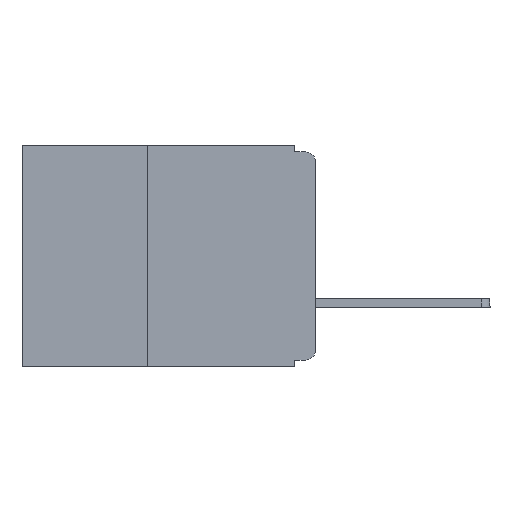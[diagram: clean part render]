
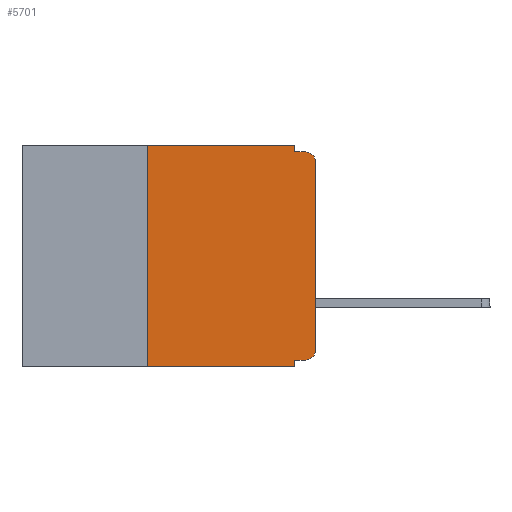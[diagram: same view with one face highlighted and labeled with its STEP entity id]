
A CAD part, left-side view. The second image highlights one B-rep face of the part: STEP entity #5701.
In plain terms, the highlighted planar face has unit normal (-1, 0, 0).
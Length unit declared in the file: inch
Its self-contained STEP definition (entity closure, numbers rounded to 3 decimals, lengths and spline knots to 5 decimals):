
#315 = CARTESIAN_POINT ( 'NONE',  ( 0., 0., -0.025 ) ) ;
#1051 = ORIENTED_EDGE ( 'NONE', *, *, #18132, .T. ) ;
#1086 = VECTOR ( 'NONE', #19033, 39.37008 ) ;
#1346 = ORIENTED_EDGE ( 'NONE', *, *, #22049, .F. ) ;
#1492 = EDGE_CURVE ( 'NONE', #18077, #1501, #22896, .T. ) ;
#1501 = VERTEX_POINT ( 'NONE', #15743 ) ;
#1744 = CIRCLE ( 'NONE', #17357, 0.015 ) ;
#1799 = VERTEX_POINT ( 'NONE', #18429 ) ;
#2339 = LINE ( 'NONE', #13697, #16317 ) ;
#2583 = VERTEX_POINT ( 'NONE', #11697 ) ;
#2683 = CARTESIAN_POINT ( 'NONE',  ( 0., 0., -0.32 ) ) ;
#2930 = LINE ( 'NONE', #21057, #21715 ) ;
#3350 = AXIS2_PLACEMENT_3D ( 'NONE', #8276, #20899, #10080 ) ;
#3381 = DIRECTION ( 'NONE',  ( 0., 0., -1. ) ) ;
#3517 = EDGE_CURVE ( 'NONE', #16970, #4614, #11600, .T. ) ;
#3595 = CARTESIAN_POINT ( 'NONE',  ( 0., 0.437, 0. ) ) ;
#3597 = ORIENTED_EDGE ( 'NONE', *, *, #13043, .T. ) ;
#4098 = LINE ( 'NONE', #2683, #18061 ) ;
#4614 = VERTEX_POINT ( 'NONE', #5202 ) ;
#4763 = DIRECTION ( 'NONE',  ( 0., -1., 0. ) ) ;
#5202 = CARTESIAN_POINT ( 'NONE',  ( 0., 0.25, 0. ) ) ;
#5456 = DIRECTION ( 'NONE',  ( 0., -1., 0. ) ) ;
#5701 = ADVANCED_FACE ( 'NONE', ( #12039 ), #13851, .F. ) ;
#5730 = DIRECTION ( 'NONE',  ( -1., 0., 0. ) ) ;
#5769 = ORIENTED_EDGE ( 'NONE', *, *, #10304, .T. ) ;
#6113 = ORIENTED_EDGE ( 'NONE', *, *, #16311, .T. ) ;
#6207 = CARTESIAN_POINT ( 'NONE',  ( 0., 0., -0.305 ) ) ;
#6278 = ORIENTED_EDGE ( 'NONE', *, *, #20713, .F. ) ;
#6481 = CARTESIAN_POINT ( 'NONE',  ( 0., 0.031, -0.01 ) ) ;
#6554 = LINE ( 'NONE', #11872, #1086 ) ;
#6602 = DIRECTION ( 'NONE',  ( 0., 0., -1. ) ) ;
#6846 = CARTESIAN_POINT ( 'NONE',  ( 0., 0.031, -0.32 ) ) ;
#7013 = CARTESIAN_POINT ( 'NONE',  ( 0., 0.25, -0.33 ) ) ;
#7179 = VECTOR ( 'NONE', #3381, 39.37008 ) ;
#8276 = CARTESIAN_POINT ( 'NONE',  ( 0., 0.015, -0.025 ) ) ;
#8500 = CARTESIAN_POINT ( 'NONE',  ( 0., 0., -0.01 ) ) ;
#8722 = CARTESIAN_POINT ( 'NONE',  ( 0., 0.25, -0.33 ) ) ;
#9146 = VERTEX_POINT ( 'NONE', #6846 ) ;
#10080 = DIRECTION ( 'NONE',  ( 0., 0., -1. ) ) ;
#10124 = ORIENTED_EDGE ( 'NONE', *, *, #1492, .F. ) ;
#10304 = EDGE_CURVE ( 'NONE', #21706, #16586, #2339, .T. ) ;
#10715 = ORIENTED_EDGE ( 'NONE', *, *, #18069, .F. ) ;
#11291 = ORIENTED_EDGE ( 'NONE', *, *, #23238, .F. ) ;
#11600 = LINE ( 'NONE', #7013, #20623 ) ;
#11697 = CARTESIAN_POINT ( 'NONE',  ( 0., 0.031, 0. ) ) ;
#11872 = CARTESIAN_POINT ( 'NONE',  ( 0., 0.031, -0.33 ) ) ;
#12020 = LINE ( 'NONE', #17890, #7179 ) ;
#12039 = FACE_OUTER_BOUND ( 'NONE', #22352, .T. ) ;
#13043 = EDGE_CURVE ( 'NONE', #18746, #21706, #1744, .T. ) ;
#13697 = CARTESIAN_POINT ( 'NONE',  ( 0., 0., 0. ) ) ;
#13851 = PLANE ( 'NONE',  #22947 ) ;
#15426 = LINE ( 'NONE', #3595, #19660 ) ;
#15502 = DIRECTION ( 'NONE',  ( 0., 0., 1. ) ) ;
#15641 = CARTESIAN_POINT ( 'NONE',  ( 0., 0.437, 0. ) ) ;
#15743 = CARTESIAN_POINT ( 'NONE',  ( 0., 0.015, -0.01 ) ) ;
#16311 = EDGE_CURVE ( 'NONE', #16586, #1501, #23461, .T. ) ;
#16317 = VECTOR ( 'NONE', #15502, 39.37008 ) ;
#16586 = VERTEX_POINT ( 'NONE', #315 ) ;
#16627 = CARTESIAN_POINT ( 'NONE',  ( 0., 0.015, -0.305 ) ) ;
#16970 = VERTEX_POINT ( 'NONE', #8722 ) ;
#17357 = AXIS2_PLACEMENT_3D ( 'NONE', #16627, #5730, #18439 ) ;
#17473 = DIRECTION ( 'NONE',  ( 1., 0., 0. ) ) ;
#17890 = CARTESIAN_POINT ( 'NONE',  ( 0., 0.031, 0. ) ) ;
#18061 = VECTOR ( 'NONE', #20830, 39.37008 ) ;
#18069 = EDGE_CURVE ( 'NONE', #18746, #9146, #4098, .T. ) ;
#18077 = VERTEX_POINT ( 'NONE', #6481 ) ;
#18132 = EDGE_CURVE ( 'NONE', #16970, #1799, #2930, .T. ) ;
#18150 = VECTOR ( 'NONE', #4763, 39.37008 ) ;
#18429 = CARTESIAN_POINT ( 'NONE',  ( 0., 0.031, -0.33 ) ) ;
#18439 = DIRECTION ( 'NONE',  ( 0., 0., -1. ) ) ;
#18746 = VERTEX_POINT ( 'NONE', #20244 ) ;
#19033 = DIRECTION ( 'NONE',  ( 0., 0., -1. ) ) ;
#19660 = VECTOR ( 'NONE', #5456, 39.37008 ) ;
#20216 = ORIENTED_EDGE ( 'NONE', *, *, #3517, .F. ) ;
#20244 = CARTESIAN_POINT ( 'NONE',  ( 0., 0.015, -0.32 ) ) ;
#20623 = VECTOR ( 'NONE', #21490, 39.37008 ) ;
#20713 = EDGE_CURVE ( 'NONE', #9146, #1799, #6554, .T. ) ;
#20830 = DIRECTION ( 'NONE',  ( 0., 1., 0. ) ) ;
#20899 = DIRECTION ( 'NONE',  ( -1., 0., 0. ) ) ;
#21057 = CARTESIAN_POINT ( 'NONE',  ( 0., 0.437, -0.33 ) ) ;
#21490 = DIRECTION ( 'NONE',  ( 0., 0., 1. ) ) ;
#21706 = VERTEX_POINT ( 'NONE', #6207 ) ;
#21715 = VECTOR ( 'NONE', #22832, 39.37008 ) ;
#22049 = EDGE_CURVE ( 'NONE', #4614, #2583, #15426, .T. ) ;
#22352 = EDGE_LOOP ( 'NONE', ( #5769, #6113, #10124, #11291, #1346, #20216, #1051, #6278, #10715, #3597 ) ) ;
#22832 = DIRECTION ( 'NONE',  ( 0., -1., 0. ) ) ;
#22896 = LINE ( 'NONE', #8500, #18150 ) ;
#22947 = AXIS2_PLACEMENT_3D ( 'NONE', #15641, #17473, #6602 ) ;
#23238 = EDGE_CURVE ( 'NONE', #2583, #18077, #12020, .T. ) ;
#23461 = CIRCLE ( 'NONE', #3350, 0.015 ) ;
